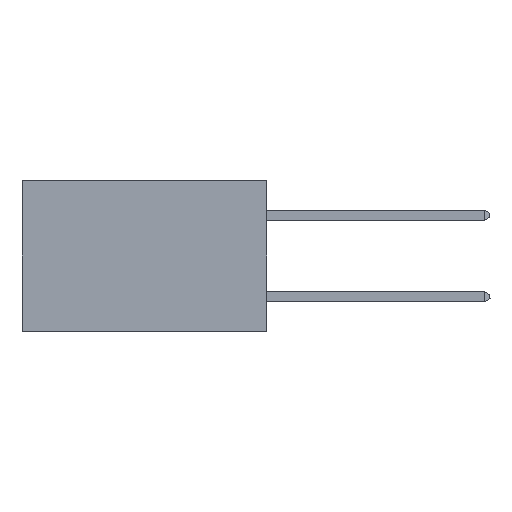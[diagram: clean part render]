
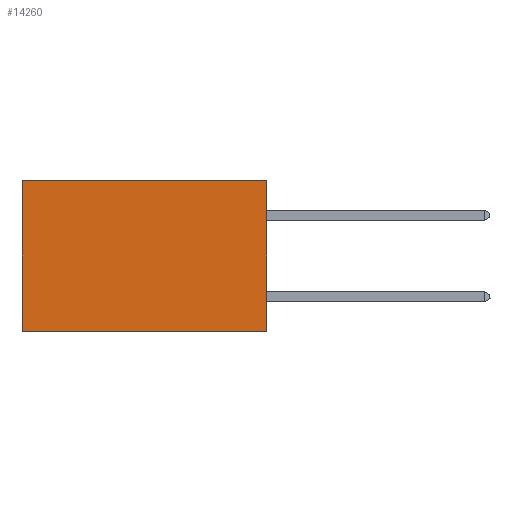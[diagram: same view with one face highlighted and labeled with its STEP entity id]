
A CAD part, left-side view. The second image highlights one B-rep face of the part: STEP entity #14260.
In plain terms, the highlighted planar face has unit normal (-1, 0, 0).
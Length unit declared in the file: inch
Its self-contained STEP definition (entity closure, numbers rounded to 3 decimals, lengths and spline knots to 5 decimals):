
#836 = VERTEX_POINT ( 'NONE', #10246 ) ;
#1911 = CARTESIAN_POINT ( 'NONE',  ( 0.2875, 0., -0.37 ) ) ;
#2292 = DIRECTION ( 'NONE',  ( 0., 0., -1. ) ) ;
#2795 = CARTESIAN_POINT ( 'NONE',  ( 0.2875, 0.6, -0.37 ) ) ;
#4127 = EDGE_CURVE ( 'NONE', #8020, #19943, #24841, .T. ) ;
#4333 = AXIS2_PLACEMENT_3D ( 'NONE', #18603, #14712, #2292 ) ;
#6811 = CARTESIAN_POINT ( 'NONE',  ( 0.2875, 0.6, 0. ) ) ;
#8020 = VERTEX_POINT ( 'NONE', #1911 ) ;
#8485 = DIRECTION ( 'NONE',  ( 0., 1., 0. ) ) ;
#8754 = VECTOR ( 'NONE', #22525, 39.37008 ) ;
#9028 = LINE ( 'NONE', #24500, #13834 ) ;
#9030 = EDGE_CURVE ( 'NONE', #836, #8020, #9028, .T. ) ;
#10246 = CARTESIAN_POINT ( 'NONE',  ( 0.2875, 0., 0. ) ) ;
#11286 = DIRECTION ( 'NONE',  ( 0., 0., -1. ) ) ;
#11379 = CARTESIAN_POINT ( 'NONE',  ( 0.2875, 0.6, 0. ) ) ;
#12922 = ORIENTED_EDGE ( 'NONE', *, *, #4127, .F. ) ;
#13067 = LINE ( 'NONE', #11379, #25727 ) ;
#13834 = VECTOR ( 'NONE', #15953, 39.37008 ) ;
#14260 = ADVANCED_FACE ( 'NONE', ( #22467 ), #24713, .F. ) ;
#14712 = DIRECTION ( 'NONE',  ( 1., 0., 0. ) ) ;
#15541 = LINE ( 'NONE', #22361, #8754 ) ;
#15953 = DIRECTION ( 'NONE',  ( 0., 0., -1. ) ) ;
#18603 = CARTESIAN_POINT ( 'NONE',  ( 0.2875, 0., 0. ) ) ;
#18882 = VERTEX_POINT ( 'NONE', #6811 ) ;
#19183 = ORIENTED_EDGE ( 'NONE', *, *, #25269, .T. ) ;
#19667 = VECTOR ( 'NONE', #8485, 39.37008 ) ;
#19681 = ORIENTED_EDGE ( 'NONE', *, *, #23510, .T. ) ;
#19943 = VERTEX_POINT ( 'NONE', #2795 ) ;
#20406 = ORIENTED_EDGE ( 'NONE', *, *, #9030, .F. ) ;
#22361 = CARTESIAN_POINT ( 'NONE',  ( 0.2875, 0., 0. ) ) ;
#22467 = FACE_OUTER_BOUND ( 'NONE', #25847, .T. ) ;
#22525 = DIRECTION ( 'NONE',  ( 0., 1., 0. ) ) ;
#22873 = CARTESIAN_POINT ( 'NONE',  ( 0.2875, 0., -0.37 ) ) ;
#23510 = EDGE_CURVE ( 'NONE', #18882, #19943, #13067, .T. ) ;
#24500 = CARTESIAN_POINT ( 'NONE',  ( 0.2875, 0., 0. ) ) ;
#24713 = PLANE ( 'NONE',  #4333 ) ;
#24841 = LINE ( 'NONE', #22873, #19667 ) ;
#25269 = EDGE_CURVE ( 'NONE', #836, #18882, #15541, .T. ) ;
#25727 = VECTOR ( 'NONE', #11286, 39.37008 ) ;
#25847 = EDGE_LOOP ( 'NONE', ( #19681, #12922, #20406, #19183 ) ) ;
